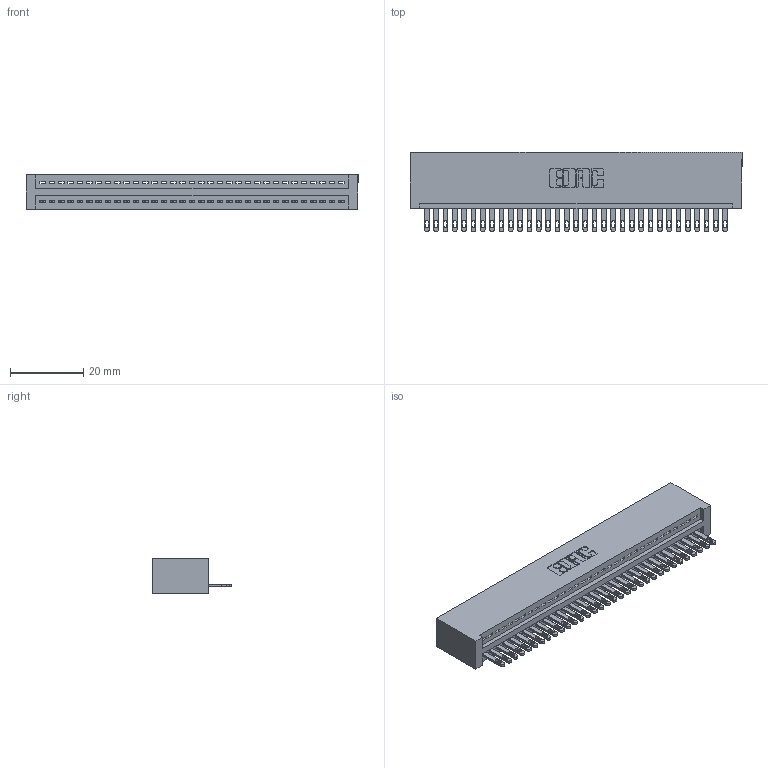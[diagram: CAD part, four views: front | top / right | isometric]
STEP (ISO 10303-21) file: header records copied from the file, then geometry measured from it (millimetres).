
FILE_DESCRIPTION (( 'STEP AP203' ), '1' );
FILE_NAME ('345-033-500-101.STEP', '2018-08-24T09:52:19', ( '' ), ( '' ), 'SwSTEP 2.0', 'SolidWorks 2016', '' );
FILE_SCHEMA (( 'CONFIG_CONTROL_DESIGN' ));
Length unit declared in the file: inch
Products named in the file (3): 345 Part_No Mounting Lugs; 345-292-001_345-293-100; 345-033-500-101
Assembly tree (34 placements, depth 2):
  345-033-500-101
    345 Part_No Mounting Lugs
    345-292-001_345-293-100  x33
Bounding box: 90.42 x 21.51 x 9.4 mm (x, y, z)
Volume: 9119.6 mm3; surface area: 12261.1 mm2
Topology: 34 solids, 34 shells, 1900 faces, 5861 edges, 3906 vertices
Faces by surface type: plane 1198, cylinder 702
Entity records: 25701 total; most frequent: CARTESIAN_POINT 4459, ORIENTED_EDGE 4426, DIRECTION 3903, EDGE_CURVE 2213, VECTOR 1953, LINE 1953, VERTEX_POINT 1474, AXIS2_PLACEMENT_3D 975
